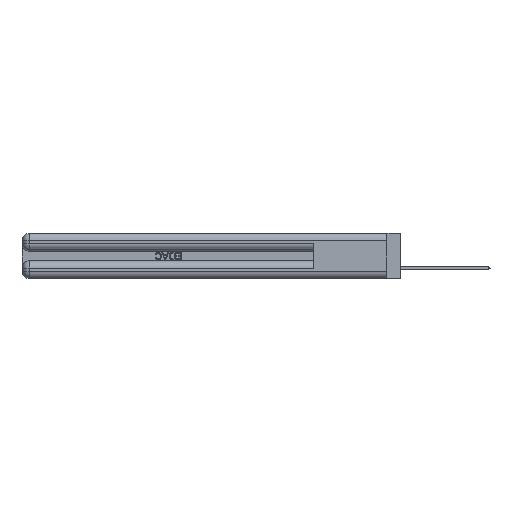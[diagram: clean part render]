
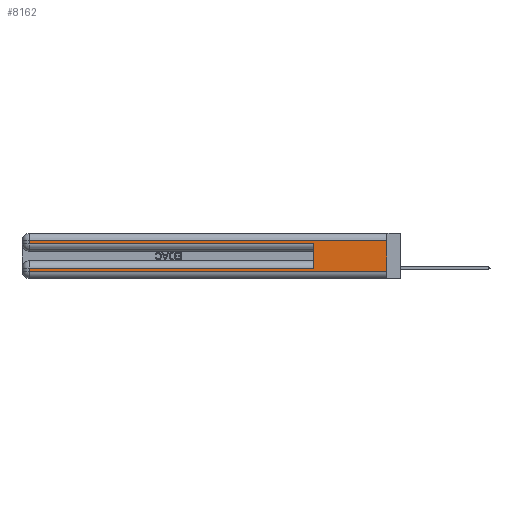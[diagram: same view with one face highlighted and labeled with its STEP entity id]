
A CAD part, left-side view. The second image highlights one B-rep face of the part: STEP entity #8162.
In plain terms, the highlighted planar face has unit normal (-1, 0, 0).
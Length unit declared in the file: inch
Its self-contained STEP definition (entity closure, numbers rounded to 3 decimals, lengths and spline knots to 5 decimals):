
#801 = CARTESIAN_POINT ( 'NONE',  ( 0., 0., 0.06 ) ) ;
#1242 = CARTESIAN_POINT ( 'NONE',  ( 0., 0., 0.285 ) ) ;
#1275 = ORIENTED_EDGE ( 'NONE', *, *, #12918, .T. ) ;
#1372 = EDGE_CURVE ( 'NONE', #11262, #26091, #20835, .T. ) ;
#2367 = CARTESIAN_POINT ( 'NONE',  ( 0., 0., 0.31 ) ) ;
#3059 = ORIENTED_EDGE ( 'NONE', *, *, #1372, .T. ) ;
#3583 = DIRECTION ( 'NONE',  ( 1., 0., 0. ) ) ;
#4154 = EDGE_LOOP ( 'NONE', ( #14158, #20362, #1275, #44646, #14886, #22414, #39040, #3059 ) ) ;
#5086 = EDGE_CURVE ( 'NONE', #41037, #15026, #47026, .T. ) ;
#5088 = CARTESIAN_POINT ( 'NONE',  ( 0., 0., 0.31 ) ) ;
#5114 = CARTESIAN_POINT ( 'NONE',  ( 0., 0., 0.06 ) ) ;
#6710 = CARTESIAN_POINT ( 'NONE',  ( 0., 2.94, 0.31 ) ) ;
#8162 = ADVANCED_FACE ( 'NONE', ( #34510 ), #10448, .F. ) ;
#8453 = DIRECTION ( 'NONE',  ( 0., 0., -1. ) ) ;
#8633 = DIRECTION ( 'NONE',  ( 0., 1., 0. ) ) ;
#10448 = PLANE ( 'NONE',  #18466 ) ;
#10977 = VECTOR ( 'NONE', #31259, 39.37008 ) ;
#11262 = VERTEX_POINT ( 'NONE', #12251 ) ;
#12251 = CARTESIAN_POINT ( 'NONE',  ( 0., 2.94, 0.06 ) ) ;
#12324 = EDGE_CURVE ( 'NONE', #42905, #37096, #28922, .T. ) ;
#12918 = EDGE_CURVE ( 'NONE', #15026, #42905, #38123, .T. ) ;
#13243 = CARTESIAN_POINT ( 'NONE',  ( 0., 0., 0.37 ) ) ;
#14008 = DIRECTION ( 'NONE',  ( 0., 0., -1. ) ) ;
#14158 = ORIENTED_EDGE ( 'NONE', *, *, #20559, .F. ) ;
#14721 = CARTESIAN_POINT ( 'NONE',  ( 0., 2.94, 0.285 ) ) ;
#14886 = ORIENTED_EDGE ( 'NONE', *, *, #44094, .F. ) ;
#15026 = VERTEX_POINT ( 'NONE', #6710 ) ;
#16639 = LINE ( 'NONE', #34122, #30537 ) ;
#17051 = CARTESIAN_POINT ( 'NONE',  ( 0., 2.94, 0.085 ) ) ;
#18048 = LINE ( 'NONE', #45124, #36052 ) ;
#18466 = AXIS2_PLACEMENT_3D ( 'NONE', #25817, #3583, #14008 ) ;
#18615 = EDGE_CURVE ( 'NONE', #23044, #33029, #16639, .T. ) ;
#19898 = DIRECTION ( 'NONE',  ( 0., -1., 0. ) ) ;
#19909 = LINE ( 'NONE', #13243, #35576 ) ;
#20362 = ORIENTED_EDGE ( 'NONE', *, *, #5086, .T. ) ;
#20559 = EDGE_CURVE ( 'NONE', #41037, #26091, #19909, .T. ) ;
#20835 = LINE ( 'NONE', #5114, #10977 ) ;
#21608 = CARTESIAN_POINT ( 'NONE',  ( 0., 0.6, 0.085 ) ) ;
#22414 = ORIENTED_EDGE ( 'NONE', *, *, #18615, .T. ) ;
#23044 = VERTEX_POINT ( 'NONE', #21608 ) ;
#23870 = LINE ( 'NONE', #34741, #34913 ) ;
#24906 = DIRECTION ( 'NONE',  ( 0., 0., -1. ) ) ;
#25817 = CARTESIAN_POINT ( 'NONE',  ( 0., 0., 0.37 ) ) ;
#26091 = VERTEX_POINT ( 'NONE', #801 ) ;
#28922 = LINE ( 'NONE', #1242, #32961 ) ;
#30537 = VECTOR ( 'NONE', #8633, 39.37008 ) ;
#31259 = DIRECTION ( 'NONE',  ( 0., -1., 0. ) ) ;
#32812 = EDGE_CURVE ( 'NONE', #33029, #11262, #23870, .T. ) ;
#32961 = VECTOR ( 'NONE', #19898, 39.37008 ) ;
#33029 = VERTEX_POINT ( 'NONE', #17051 ) ;
#34122 = CARTESIAN_POINT ( 'NONE',  ( 0., 0., 0.085 ) ) ;
#34510 = FACE_OUTER_BOUND ( 'NONE', #4154, .T. ) ;
#34741 = CARTESIAN_POINT ( 'NONE',  ( 0., 2.94, 0.37 ) ) ;
#34913 = VECTOR ( 'NONE', #8453, 39.37008 ) ;
#35212 = VECTOR ( 'NONE', #43554, 39.37008 ) ;
#35576 = VECTOR ( 'NONE', #24906, 39.37008 ) ;
#36052 = VECTOR ( 'NONE', #40936, 39.37008 ) ;
#37096 = VERTEX_POINT ( 'NONE', #44412 ) ;
#38123 = LINE ( 'NONE', #46284, #35212 ) ;
#39021 = DIRECTION ( 'NONE',  ( 0., 1., 0. ) ) ;
#39040 = ORIENTED_EDGE ( 'NONE', *, *, #32812, .T. ) ;
#40936 = DIRECTION ( 'NONE',  ( 0., 0., 1. ) ) ;
#41037 = VERTEX_POINT ( 'NONE', #5088 ) ;
#42905 = VERTEX_POINT ( 'NONE', #14721 ) ;
#42937 = VECTOR ( 'NONE', #39021, 39.37008 ) ;
#43554 = DIRECTION ( 'NONE',  ( 0., 0., -1. ) ) ;
#44094 = EDGE_CURVE ( 'NONE', #23044, #37096, #18048, .T. ) ;
#44412 = CARTESIAN_POINT ( 'NONE',  ( 0., 0.6, 0.285 ) ) ;
#44646 = ORIENTED_EDGE ( 'NONE', *, *, #12324, .T. ) ;
#45124 = CARTESIAN_POINT ( 'NONE',  ( 0., 0.6, 0.145 ) ) ;
#46284 = CARTESIAN_POINT ( 'NONE',  ( 0., 2.94, 0.37 ) ) ;
#47026 = LINE ( 'NONE', #2367, #42937 ) ;
